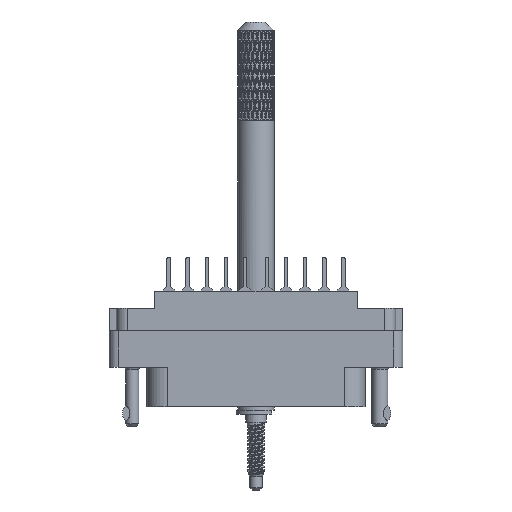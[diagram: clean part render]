
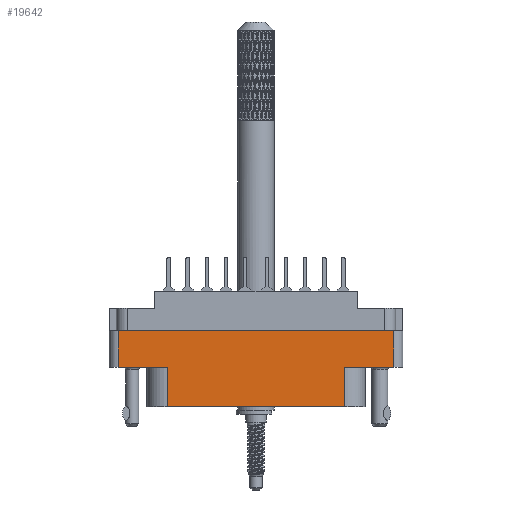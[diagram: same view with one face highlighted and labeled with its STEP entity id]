
A CAD part, front view. The second image highlights one B-rep face of the part: STEP entity #19642.
In plain terms, the highlighted planar face has unit normal (0, -1, 0).
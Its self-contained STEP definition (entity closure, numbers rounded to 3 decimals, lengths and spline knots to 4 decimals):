
#2762 = CARTESIAN_POINT ( 'NONE',  ( -0.938, -0.438, -0.268 ) ) ;
#3047 = EDGE_CURVE ( 'NONE', #40710, #49875, #85124, .T. ) ;
#5696 = DIRECTION ( 'NONE',  ( 1., 0., 0. ) ) ;
#6101 = VERTEX_POINT ( 'NONE', #24639 ) ;
#6195 = CARTESIAN_POINT ( 'NONE',  ( 0.604, -0.438, -0.52 ) ) ;
#6576 = CARTESIAN_POINT ( 'NONE',  ( 0., -0.438, -0.268 ) ) ;
#9925 = CARTESIAN_POINT ( 'NONE',  ( -0.604, -0.438, -0.52 ) ) ;
#10737 = ORIENTED_EDGE ( 'NONE', *, *, #95545, .T. ) ;
#12835 = DIRECTION ( 'NONE',  ( 0., -1., 0. ) ) ;
#15970 = ORIENTED_EDGE ( 'NONE', *, *, #39735, .F. ) ;
#16365 = ORIENTED_EDGE ( 'NONE', *, *, #31241, .F. ) ;
#16534 = VECTOR ( 'NONE', #50380, 39.3701 ) ;
#17600 = FACE_OUTER_BOUND ( 'NONE', #74537, .T. ) ;
#18121 = CARTESIAN_POINT ( 'NONE',  ( 0.604, -0.438, -0.52 ) ) ;
#18123 = EDGE_CURVE ( 'NONE', #49875, #55803, #38175, .T. ) ;
#19642 = ADVANCED_FACE ( 'NONE', ( #17600 ), #99482, .T. ) ;
#20145 = LINE ( 'NONE', #23489, #88206 ) ;
#21796 = VECTOR ( 'NONE', #36577, 39.3701 ) ;
#23489 = CARTESIAN_POINT ( 'NONE',  ( 0.938, -0.438, -0.789 ) ) ;
#23815 = ORIENTED_EDGE ( 'NONE', *, *, #100967, .T. ) ;
#24639 = CARTESIAN_POINT ( 'NONE',  ( 0.938, -0.438, -0.268 ) ) ;
#26230 = LINE ( 'NONE', #6195, #95580 ) ;
#27431 = DIRECTION ( 'NONE',  ( -1., 0., 0. ) ) ;
#28552 = CARTESIAN_POINT ( 'NONE',  ( -0.938, -0.438, -0.789 ) ) ;
#30826 = CARTESIAN_POINT ( 'NONE',  ( -1., -0.438, -0.789 ) ) ;
#31241 = EDGE_CURVE ( 'NONE', #88548, #6101, #39623, .T. ) ;
#35090 = CARTESIAN_POINT ( 'NONE',  ( -0.938, -0.438, -0.52 ) ) ;
#36577 = DIRECTION ( 'NONE',  ( 0., 0., -1. ) ) ;
#38175 = LINE ( 'NONE', #77272, #21796 ) ;
#39623 = LINE ( 'NONE', #6576, #16534 ) ;
#39735 = EDGE_CURVE ( 'NONE', #100684, #101636, #112136, .T. ) ;
#40710 = VERTEX_POINT ( 'NONE', #35090 ) ;
#46020 = VECTOR ( 'NONE', #90512, 39.3701 ) ;
#47532 = CARTESIAN_POINT ( 'NONE',  ( 0.938, -0.438, -0.52 ) ) ;
#49875 = VERTEX_POINT ( 'NONE', #9925 ) ;
#50006 = EDGE_CURVE ( 'NONE', #88548, #40710, #90820, .T. ) ;
#50286 = DIRECTION ( 'NONE',  ( 1., 0., 0. ) ) ;
#50380 = DIRECTION ( 'NONE',  ( 1., 0., 0. ) ) ;
#53352 = LINE ( 'NONE', #30826, #102222 ) ;
#53896 = VECTOR ( 'NONE', #50286, 39.3701 ) ;
#54298 = VERTEX_POINT ( 'NONE', #74129 ) ;
#55803 = VERTEX_POINT ( 'NONE', #76502 ) ;
#57049 = DIRECTION ( 'NONE',  ( 0., 0., -1. ) ) ;
#59155 = ORIENTED_EDGE ( 'NONE', *, *, #3047, .T. ) ;
#62226 = EDGE_CURVE ( 'NONE', #54298, #101636, #26230, .T. ) ;
#63331 = AXIS2_PLACEMENT_3D ( 'NONE', #82416, #12835, #57049 ) ;
#63532 = ORIENTED_EDGE ( 'NONE', *, *, #18123, .T. ) ;
#65857 = CARTESIAN_POINT ( 'NONE',  ( 0., -0.438, -0.52 ) ) ;
#69371 = DIRECTION ( 'NONE',  ( 0., 0., 1. ) ) ;
#70781 = CARTESIAN_POINT ( 'NONE',  ( 0., -0.438, -0.52 ) ) ;
#74129 = CARTESIAN_POINT ( 'NONE',  ( 0.604, -0.438, -0.789 ) ) ;
#74537 = EDGE_LOOP ( 'NONE', ( #16365, #107125, #59155, #63532, #10737, #101073, #15970, #23815 ) ) ;
#76502 = CARTESIAN_POINT ( 'NONE',  ( -0.604, -0.438, -0.789 ) ) ;
#77272 = CARTESIAN_POINT ( 'NONE',  ( -0.604, -0.438, -0.789 ) ) ;
#82416 = CARTESIAN_POINT ( 'NONE',  ( -1., -0.438, -0.789 ) ) ;
#85124 = LINE ( 'NONE', #65857, #53896 ) ;
#88206 = VECTOR ( 'NONE', #99342, 39.3701 ) ;
#88548 = VERTEX_POINT ( 'NONE', #2762 ) ;
#90512 = DIRECTION ( 'NONE',  ( 0., 0., -1. ) ) ;
#90820 = LINE ( 'NONE', #28552, #46020 ) ;
#95545 = EDGE_CURVE ( 'NONE', #55803, #54298, #53352, .T. ) ;
#95580 = VECTOR ( 'NONE', #69371, 39.3701 ) ;
#97246 = VECTOR ( 'NONE', #27431, 39.3701 ) ;
#99342 = DIRECTION ( 'NONE',  ( 0., 0., 1. ) ) ;
#99482 = PLANE ( 'NONE',  #63331 ) ;
#100684 = VERTEX_POINT ( 'NONE', #47532 ) ;
#100967 = EDGE_CURVE ( 'NONE', #100684, #6101, #20145, .T. ) ;
#101073 = ORIENTED_EDGE ( 'NONE', *, *, #62226, .T. ) ;
#101636 = VERTEX_POINT ( 'NONE', #18121 ) ;
#102222 = VECTOR ( 'NONE', #5696, 39.3701 ) ;
#107125 = ORIENTED_EDGE ( 'NONE', *, *, #50006, .T. ) ;
#112136 = LINE ( 'NONE', #70781, #97246 ) ;
